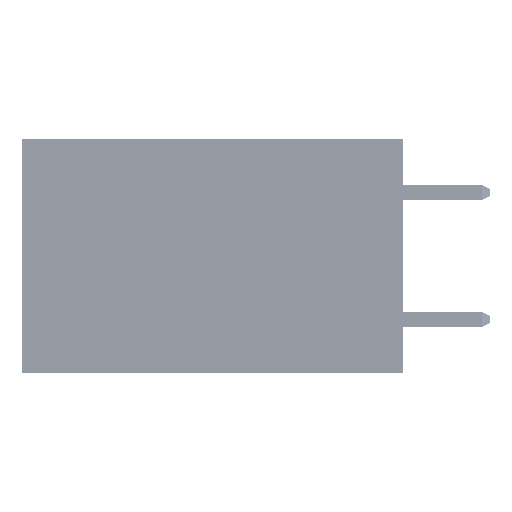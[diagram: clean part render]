
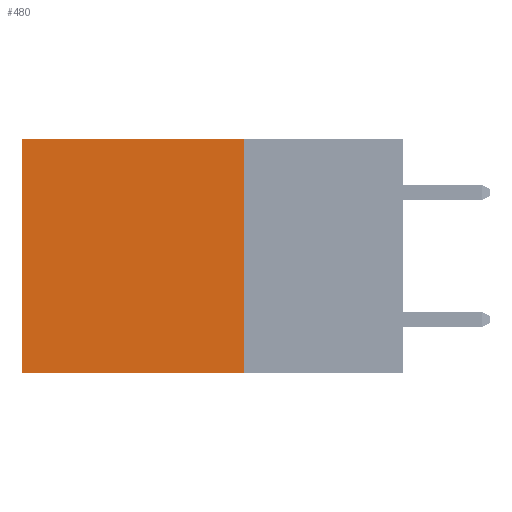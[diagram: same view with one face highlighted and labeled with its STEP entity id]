
A CAD part, left-side view. The second image highlights one B-rep face of the part: STEP entity #480.
In plain terms, the highlighted planar face has unit normal (-1, 0, 0).
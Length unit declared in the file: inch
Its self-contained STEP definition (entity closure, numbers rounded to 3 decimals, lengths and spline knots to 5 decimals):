
#480 = ADVANCED_FACE ( 'NONE', ( #29139 ), #35165, .F. ) ;
#3459 = VERTEX_POINT ( 'NONE', #15454 ) ;
#4611 = VECTOR ( 'NONE', #37501, 39.37008 ) ;
#5191 = CARTESIAN_POINT ( 'NONE',  ( 0.2875, 0.25, 0. ) ) ;
#8746 = CARTESIAN_POINT ( 'NONE',  ( 0.2875, 0.25, 0. ) ) ;
#11247 = ORIENTED_EDGE ( 'NONE', *, *, #43995, .F. ) ;
#14382 = CARTESIAN_POINT ( 'NONE',  ( 0.2875, 0.6, 0. ) ) ;
#14813 = CARTESIAN_POINT ( 'NONE',  ( 0.2875, 0.6, -0.37 ) ) ;
#15454 = CARTESIAN_POINT ( 'NONE',  ( 0.2875, 0.6, 0. ) ) ;
#16543 = DIRECTION ( 'NONE',  ( 0., 1., 0. ) ) ;
#17260 = DIRECTION ( 'NONE',  ( 0., 0., -1. ) ) ;
#17889 = EDGE_CURVE ( 'NONE', #36315, #41779, #33262, .T. ) ;
#18027 = DIRECTION ( 'NONE',  ( 0., 0., -1. ) ) ;
#19478 = EDGE_CURVE ( 'NONE', #3459, #26520, #22482, .T. ) ;
#19509 = ORIENTED_EDGE ( 'NONE', *, *, #19478, .T. ) ;
#20938 = EDGE_CURVE ( 'NONE', #36315, #3459, #44329, .T. ) ;
#21173 = DIRECTION ( 'NONE',  ( 0., 1., 0. ) ) ;
#22482 = LINE ( 'NONE', #14382, #40509 ) ;
#23057 = EDGE_LOOP ( 'NONE', ( #19509, #11247, #32867, #37799 ) ) ;
#23456 = VECTOR ( 'NONE', #16543, 39.37008 ) ;
#25131 = VECTOR ( 'NONE', #21173, 39.37008 ) ;
#26520 = VERTEX_POINT ( 'NONE', #14813 ) ;
#27922 = CARTESIAN_POINT ( 'NONE',  ( 0.2875, 0.25, 0. ) ) ;
#28385 = CARTESIAN_POINT ( 'NONE',  ( 0.2875, 0.25, 0. ) ) ;
#29139 = FACE_OUTER_BOUND ( 'NONE', #23057, .T. ) ;
#32760 = AXIS2_PLACEMENT_3D ( 'NONE', #27922, #38806, #17260 ) ;
#32867 = ORIENTED_EDGE ( 'NONE', *, *, #17889, .F. ) ;
#33188 = CARTESIAN_POINT ( 'NONE',  ( 0.2875, 0.25, -0.37 ) ) ;
#33262 = LINE ( 'NONE', #8746, #4611 ) ;
#35165 = PLANE ( 'NONE',  #32760 ) ;
#36315 = VERTEX_POINT ( 'NONE', #5191 ) ;
#37501 = DIRECTION ( 'NONE',  ( 0., 0., -1. ) ) ;
#37799 = ORIENTED_EDGE ( 'NONE', *, *, #20938, .T. ) ;
#38806 = DIRECTION ( 'NONE',  ( 1., 0., 0. ) ) ;
#40509 = VECTOR ( 'NONE', #18027, 39.37008 ) ;
#41710 = CARTESIAN_POINT ( 'NONE',  ( 0.2875, 0.25, -0.37 ) ) ;
#41779 = VERTEX_POINT ( 'NONE', #33188 ) ;
#42627 = LINE ( 'NONE', #41710, #23456 ) ;
#43995 = EDGE_CURVE ( 'NONE', #41779, #26520, #42627, .T. ) ;
#44329 = LINE ( 'NONE', #28385, #25131 ) ;
